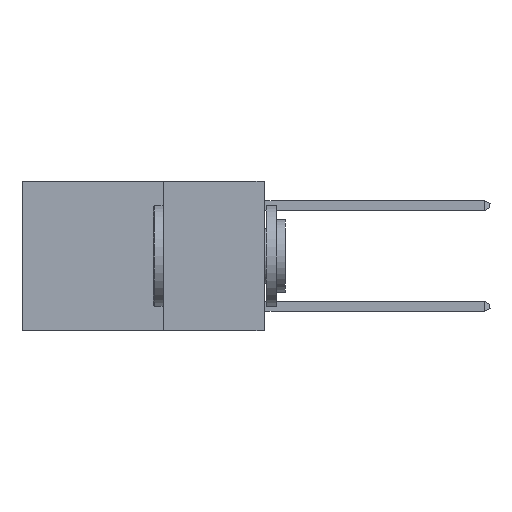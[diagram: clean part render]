
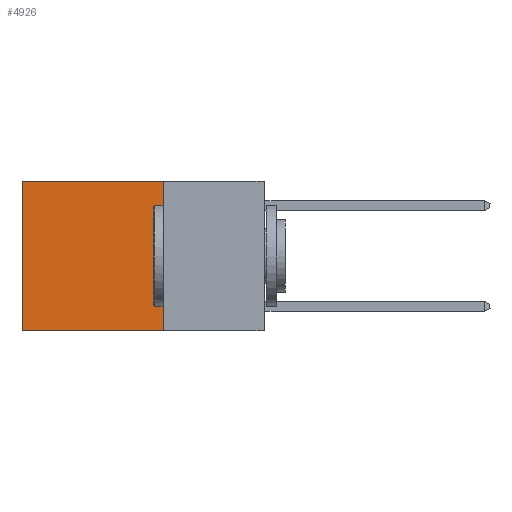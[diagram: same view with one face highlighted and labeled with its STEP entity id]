
A CAD part, left-side view. The second image highlights one B-rep face of the part: STEP entity #4926.
In plain terms, the highlighted planar face has unit normal (-1, 0, 0).
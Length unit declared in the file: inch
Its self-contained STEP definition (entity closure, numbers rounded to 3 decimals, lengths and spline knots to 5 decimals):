
#262 = CARTESIAN_POINT ( 'NONE',  ( 0.2625, 0.25, 0. ) ) ;
#1218 = LINE ( 'NONE', #12529, #10757 ) ;
#1265 = VERTEX_POINT ( 'NONE', #262 ) ;
#1519 = VERTEX_POINT ( 'NONE', #9862 ) ;
#1750 = DIRECTION ( 'NONE',  ( 0., 0., -1. ) ) ;
#1811 = VERTEX_POINT ( 'NONE', #7127 ) ;
#2106 = VERTEX_POINT ( 'NONE', #3568 ) ;
#2537 = VECTOR ( 'NONE', #11677, 39.37008 ) ;
#2684 = PLANE ( 'NONE',  #3605 ) ;
#3568 = CARTESIAN_POINT ( 'NONE',  ( 0.2625, 0.6, 0. ) ) ;
#3605 = AXIS2_PLACEMENT_3D ( 'NONE', #7096, #11662, #1750 ) ;
#3611 = ORIENTED_EDGE ( 'NONE', *, *, #11030, .F. ) ;
#3932 = ORIENTED_EDGE ( 'NONE', *, *, #8721, .T. ) ;
#4048 = DIRECTION ( 'NONE',  ( 0., 0., -1. ) ) ;
#4335 = LINE ( 'NONE', #7499, #11229 ) ;
#4926 = ADVANCED_FACE ( 'NONE', ( #6074 ), #2684, .F. ) ;
#5262 = EDGE_LOOP ( 'NONE', ( #3932, #8831, #3611, #6552 ) ) ;
#5840 = DIRECTION ( 'NONE',  ( 0., 1., 0. ) ) ;
#6074 = FACE_OUTER_BOUND ( 'NONE', #5262, .T. ) ;
#6392 = CARTESIAN_POINT ( 'NONE',  ( 0.2625, 0.6, 0. ) ) ;
#6552 = ORIENTED_EDGE ( 'NONE', *, *, #13207, .T. ) ;
#7096 = CARTESIAN_POINT ( 'NONE',  ( 0.2625, 0.25, 0. ) ) ;
#7127 = CARTESIAN_POINT ( 'NONE',  ( 0.2625, 0.25, -0.37 ) ) ;
#7499 = CARTESIAN_POINT ( 'NONE',  ( 0.2625, 0.25, 0. ) ) ;
#8721 = EDGE_CURVE ( 'NONE', #2106, #1519, #14290, .T. ) ;
#8831 = ORIENTED_EDGE ( 'NONE', *, *, #12531, .F. ) ;
#9862 = CARTESIAN_POINT ( 'NONE',  ( 0.2625, 0.6, -0.37 ) ) ;
#10757 = VECTOR ( 'NONE', #5840, 39.37008 ) ;
#10941 = VECTOR ( 'NONE', #4048, 39.37008 ) ;
#11030 = EDGE_CURVE ( 'NONE', #1265, #1811, #12859, .T. ) ;
#11229 = VECTOR ( 'NONE', #11848, 39.37008 ) ;
#11662 = DIRECTION ( 'NONE',  ( 1., 0., 0. ) ) ;
#11677 = DIRECTION ( 'NONE',  ( 0., 0., -1. ) ) ;
#11848 = DIRECTION ( 'NONE',  ( 0., 1., 0. ) ) ;
#12529 = CARTESIAN_POINT ( 'NONE',  ( 0.2625, 0.25, -0.37 ) ) ;
#12531 = EDGE_CURVE ( 'NONE', #1811, #1519, #1218, .T. ) ;
#12859 = LINE ( 'NONE', #13010, #2537 ) ;
#13010 = CARTESIAN_POINT ( 'NONE',  ( 0.2625, 0.25, 0. ) ) ;
#13207 = EDGE_CURVE ( 'NONE', #1265, #2106, #4335, .T. ) ;
#14290 = LINE ( 'NONE', #6392, #10941 ) ;
